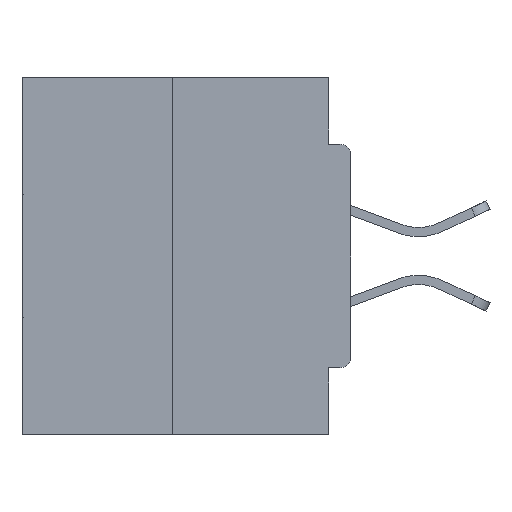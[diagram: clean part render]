
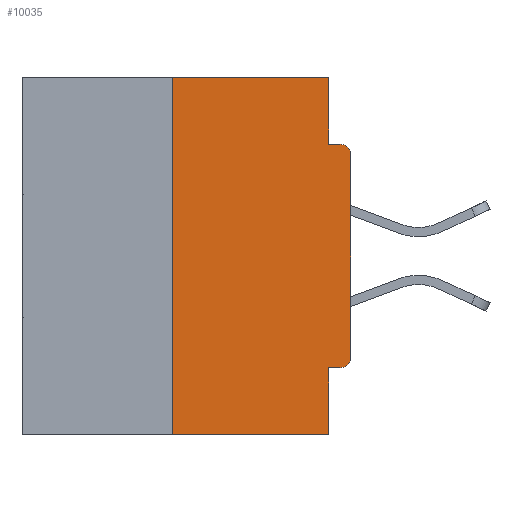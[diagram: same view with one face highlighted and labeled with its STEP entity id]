
A CAD part, left-side view. The second image highlights one B-rep face of the part: STEP entity #10035.
In plain terms, the highlighted planar face has unit normal (-1, 0, 0).
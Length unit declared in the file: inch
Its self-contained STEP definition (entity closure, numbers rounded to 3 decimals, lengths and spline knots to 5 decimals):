
#76 = DIRECTION ( 'NONE',  ( -1., 0., 0. ) ) ;
#447 = ORIENTED_EDGE ( 'NONE', *, *, #29793, .T. ) ;
#554 = VERTEX_POINT ( 'NONE', #13984 ) ;
#828 = LINE ( 'NONE', #19448, #17412 ) ;
#867 = AXIS2_PLACEMENT_3D ( 'NONE', #17820, #76, #11621 ) ;
#1224 = CARTESIAN_POINT ( 'NONE',  ( 0., 0.015, -0.0935 ) ) ;
#2035 = CARTESIAN_POINT ( 'NONE',  ( 0., 0., -0.0935 ) ) ;
#2043 = VECTOR ( 'NONE', #9806, 39.37008 ) ;
#2235 = CARTESIAN_POINT ( 'NONE',  ( 0., 0.25, 0. ) ) ;
#2337 = AXIS2_PLACEMENT_3D ( 'NONE', #6723, #9512, #15692 ) ;
#3678 = CARTESIAN_POINT ( 'NONE',  ( 0., 0.031, -0.5 ) ) ;
#3717 = VERTEX_POINT ( 'NONE', #12065 ) ;
#4292 = EDGE_CURVE ( 'NONE', #14212, #30719, #35158, .T. ) ;
#4323 = AXIS2_PLACEMENT_3D ( 'NONE', #15855, #13069, #7266 ) ;
#4478 = EDGE_CURVE ( 'NONE', #16884, #30719, #23354, .T. ) ;
#5018 = DIRECTION ( 'NONE',  ( 0., 0., -1. ) ) ;
#5283 = CARTESIAN_POINT ( 'NONE',  ( 0., 0.015, -0.4065 ) ) ;
#5427 = ORIENTED_EDGE ( 'NONE', *, *, #35150, .T. ) ;
#5524 = ORIENTED_EDGE ( 'NONE', *, *, #28375, .F. ) ;
#5602 = ORIENTED_EDGE ( 'NONE', *, *, #17707, .F. ) ;
#6723 = CARTESIAN_POINT ( 'NONE',  ( 0., 0.015, -0.3915 ) ) ;
#7107 = DIRECTION ( 'NONE',  ( 0., -1., 0. ) ) ;
#7141 = CARTESIAN_POINT ( 'NONE',  ( 0., 0.25, 0. ) ) ;
#7266 = DIRECTION ( 'NONE',  ( 0., 0., -1. ) ) ;
#7709 = CARTESIAN_POINT ( 'NONE',  ( 0., 0., -0.4065 ) ) ;
#9512 = DIRECTION ( 'NONE',  ( -1., 0., 0. ) ) ;
#9806 = DIRECTION ( 'NONE',  ( 0., 0., -1. ) ) ;
#10035 = ADVANCED_FACE ( 'NONE', ( #15706 ), #31177, .F. ) ;
#10288 = ORIENTED_EDGE ( 'NONE', *, *, #4292, .T. ) ;
#11621 = DIRECTION ( 'NONE',  ( 0., 0., -1. ) ) ;
#12065 = CARTESIAN_POINT ( 'NONE',  ( 0., 0., -0.1085 ) ) ;
#13069 = DIRECTION ( 'NONE',  ( 1., 0., 0. ) ) ;
#13275 = ORIENTED_EDGE ( 'NONE', *, *, #16909, .F. ) ;
#13645 = VECTOR ( 'NONE', #17279, 39.37008 ) ;
#13660 = DIRECTION ( 'NONE',  ( 0., -1., 0. ) ) ;
#13889 = EDGE_CURVE ( 'NONE', #37757, #28752, #828, .T. ) ;
#13984 = CARTESIAN_POINT ( 'NONE',  ( 0., 0., -0.3915 ) ) ;
#14212 = VERTEX_POINT ( 'NONE', #25237 ) ;
#15692 = DIRECTION ( 'NONE',  ( 0., 0., -1. ) ) ;
#15706 = FACE_OUTER_BOUND ( 'NONE', #30261, .T. ) ;
#15855 = CARTESIAN_POINT ( 'NONE',  ( 0., 0.46, 0. ) ) ;
#16230 = DIRECTION ( 'NONE',  ( 0., 0., 1. ) ) ;
#16768 = ORIENTED_EDGE ( 'NONE', *, *, #13889, .F. ) ;
#16884 = VERTEX_POINT ( 'NONE', #19556 ) ;
#16909 = EDGE_CURVE ( 'NONE', #30491, #16884, #37436, .T. ) ;
#17256 = VERTEX_POINT ( 'NONE', #17269 ) ;
#17269 = CARTESIAN_POINT ( 'NONE',  ( 0., 0.031, -0.0935 ) ) ;
#17279 = DIRECTION ( 'NONE',  ( 0., 0., 1. ) ) ;
#17412 = VECTOR ( 'NONE', #13660, 39.37008 ) ;
#17707 = EDGE_CURVE ( 'NONE', #14212, #37757, #19619, .T. ) ;
#17820 = CARTESIAN_POINT ( 'NONE',  ( 0., 0.015, -0.1085 ) ) ;
#18890 = ORIENTED_EDGE ( 'NONE', *, *, #36498, .T. ) ;
#19448 = CARTESIAN_POINT ( 'NONE',  ( 0., 0.46, 0. ) ) ;
#19556 = CARTESIAN_POINT ( 'NONE',  ( 0., 0.031, -0.4065 ) ) ;
#19619 = LINE ( 'NONE', #7141, #38514 ) ;
#20457 = ORIENTED_EDGE ( 'NONE', *, *, #38191, .F. ) ;
#21171 = LINE ( 'NONE', #31983, #23037 ) ;
#23037 = VECTOR ( 'NONE', #5018, 39.37008 ) ;
#23110 = LINE ( 'NONE', #32329, #13645 ) ;
#23354 = LINE ( 'NONE', #3678, #2043 ) ;
#24038 = VECTOR ( 'NONE', #38814, 39.37008 ) ;
#24562 = CARTESIAN_POINT ( 'NONE',  ( 0., 0.031, -0.5 ) ) ;
#25237 = CARTESIAN_POINT ( 'NONE',  ( 0., 0.25, -0.5 ) ) ;
#25314 = CARTESIAN_POINT ( 'NONE',  ( 0., 0.031, 0. ) ) ;
#26136 = VECTOR ( 'NONE', #31739, 39.37008 ) ;
#28375 = EDGE_CURVE ( 'NONE', #17256, #29947, #33498, .T. ) ;
#28752 = VERTEX_POINT ( 'NONE', #25314 ) ;
#29793 = EDGE_CURVE ( 'NONE', #30491, #554, #35312, .T. ) ;
#29947 = VERTEX_POINT ( 'NONE', #1224 ) ;
#30045 = ORIENTED_EDGE ( 'NONE', *, *, #4478, .F. ) ;
#30261 = EDGE_LOOP ( 'NONE', ( #16768, #5602, #10288, #30045, #13275, #447, #5427, #18890, #5524, #20457 ) ) ;
#30491 = VERTEX_POINT ( 'NONE', #5283 ) ;
#30719 = VERTEX_POINT ( 'NONE', #24562 ) ;
#31177 = PLANE ( 'NONE',  #4323 ) ;
#31739 = DIRECTION ( 'NONE',  ( 0., 1., 0. ) ) ;
#31983 = CARTESIAN_POINT ( 'NONE',  ( 0., 0.031, 0. ) ) ;
#32329 = CARTESIAN_POINT ( 'NONE',  ( 0., 0., 0. ) ) ;
#32336 = VECTOR ( 'NONE', #7107, 39.37008 ) ;
#33498 = LINE ( 'NONE', #2035, #24038 ) ;
#33895 = CARTESIAN_POINT ( 'NONE',  ( 0., 0.46, -0.5 ) ) ;
#35150 = EDGE_CURVE ( 'NONE', #554, #3717, #23110, .T. ) ;
#35158 = LINE ( 'NONE', #33895, #32336 ) ;
#35312 = CIRCLE ( 'NONE', #2337, 0.015 ) ;
#36498 = EDGE_CURVE ( 'NONE', #3717, #29947, #37844, .T. ) ;
#37436 = LINE ( 'NONE', #7709, #26136 ) ;
#37757 = VERTEX_POINT ( 'NONE', #2235 ) ;
#37844 = CIRCLE ( 'NONE', #867, 0.015 ) ;
#38191 = EDGE_CURVE ( 'NONE', #28752, #17256, #21171, .T. ) ;
#38514 = VECTOR ( 'NONE', #16230, 39.37008 ) ;
#38814 = DIRECTION ( 'NONE',  ( 0., -1., 0. ) ) ;
